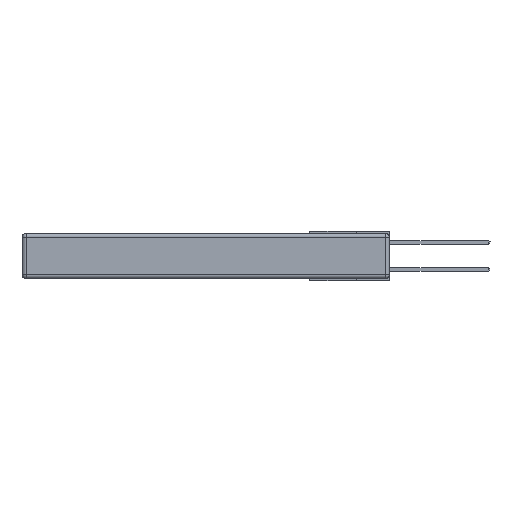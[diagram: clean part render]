
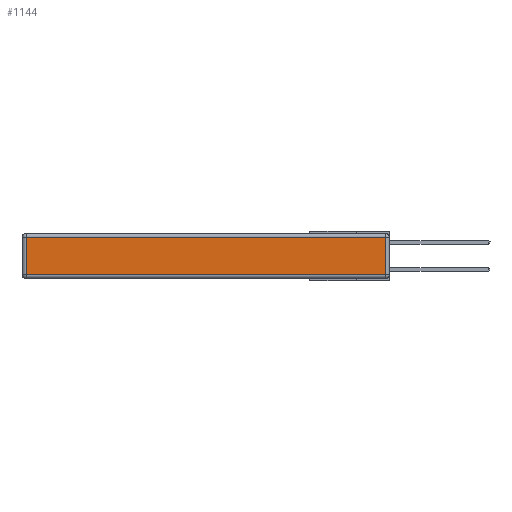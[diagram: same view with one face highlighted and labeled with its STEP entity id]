
A CAD part, left-side view. The second image highlights one B-rep face of the part: STEP entity #1144.
In plain terms, the highlighted planar face has unit normal (-1, 0, 0).
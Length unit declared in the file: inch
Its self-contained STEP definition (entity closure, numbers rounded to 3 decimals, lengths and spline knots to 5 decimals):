
#250 = VERTEX_POINT ( 'NONE', #20595 ) ;
#652 = VERTEX_POINT ( 'NONE', #22547 ) ;
#1144 = ADVANCED_FACE ( 'NONE', ( #26830 ), #28529, .T. ) ;
#2948 = DIRECTION ( 'NONE',  ( -1., 0., 0. ) ) ;
#4426 = VERTEX_POINT ( 'NONE', #16344 ) ;
#8546 = VERTEX_POINT ( 'NONE', #27394 ) ;
#8819 = ORIENTED_EDGE ( 'NONE', *, *, #22804, .T. ) ;
#10647 = EDGE_LOOP ( 'NONE', ( #17229, #26781, #21161, #8819 ) ) ;
#11267 = VECTOR ( 'NONE', #23400, 39.37008 ) ;
#13146 = LINE ( 'NONE', #21869, #21164 ) ;
#13309 = LINE ( 'NONE', #24193, #22051 ) ;
#14678 = DIRECTION ( 'NONE',  ( 0., 0., 1. ) ) ;
#16344 = CARTESIAN_POINT ( 'NONE',  ( 0., 0.03, -0.313 ) ) ;
#16351 = VECTOR ( 'NONE', #27903, 39.37008 ) ;
#16948 = CARTESIAN_POINT ( 'NONE',  ( 0., 0., -0.343 ) ) ;
#17126 = EDGE_CURVE ( 'NONE', #250, #652, #18937, .T. ) ;
#17229 = ORIENTED_EDGE ( 'NONE', *, *, #27578, .T. ) ;
#17883 = DIRECTION ( 'NONE',  ( 0., 0., -1. ) ) ;
#18937 = LINE ( 'NONE', #25478, #16351 ) ;
#19088 = CARTESIAN_POINT ( 'NONE',  ( 0., 0., -0.313 ) ) ;
#19825 = DIRECTION ( 'NONE',  ( 0., 0., 1. ) ) ;
#20595 = CARTESIAN_POINT ( 'NONE',  ( 0., 0.03, -0.03 ) ) ;
#21161 = ORIENTED_EDGE ( 'NONE', *, *, #17126, .T. ) ;
#21164 = VECTOR ( 'NONE', #17883, 39.37008 ) ;
#21869 = CARTESIAN_POINT ( 'NONE',  ( 0., 2.72, -0.343 ) ) ;
#22051 = VECTOR ( 'NONE', #19825, 39.37008 ) ;
#22547 = CARTESIAN_POINT ( 'NONE',  ( 0., 2.72, -0.03 ) ) ;
#22804 = EDGE_CURVE ( 'NONE', #652, #8546, #13146, .T. ) ;
#23264 = LINE ( 'NONE', #19088, #11267 ) ;
#23400 = DIRECTION ( 'NONE',  ( 0., -1., 0. ) ) ;
#23751 = AXIS2_PLACEMENT_3D ( 'NONE', #16948, #2948, #14678 ) ;
#24193 = CARTESIAN_POINT ( 'NONE',  ( 0., 0.03, -0.343 ) ) ;
#25478 = CARTESIAN_POINT ( 'NONE',  ( 0., 2.75, -0.03 ) ) ;
#25614 = EDGE_CURVE ( 'NONE', #4426, #250, #13309, .T. ) ;
#26781 = ORIENTED_EDGE ( 'NONE', *, *, #25614, .T. ) ;
#26830 = FACE_OUTER_BOUND ( 'NONE', #10647, .T. ) ;
#27394 = CARTESIAN_POINT ( 'NONE',  ( 0., 2.72, -0.313 ) ) ;
#27578 = EDGE_CURVE ( 'NONE', #8546, #4426, #23264, .T. ) ;
#27903 = DIRECTION ( 'NONE',  ( 0., 1., 0. ) ) ;
#28529 = PLANE ( 'NONE',  #23751 ) ;
